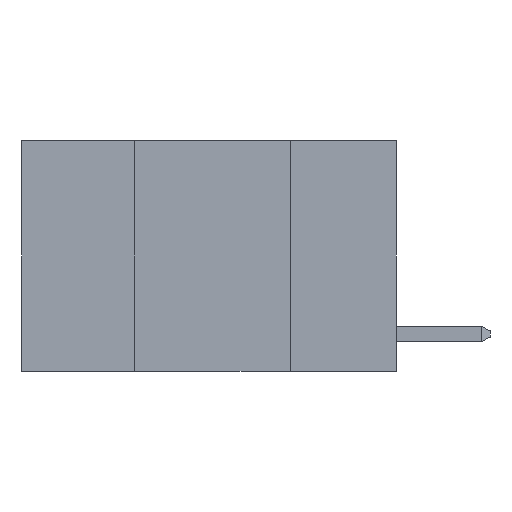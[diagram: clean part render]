
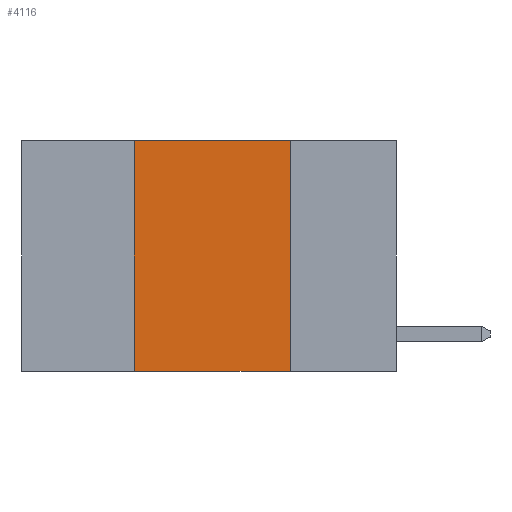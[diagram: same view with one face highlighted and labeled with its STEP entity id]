
A CAD part, left-side view. The second image highlights one B-rep face of the part: STEP entity #4116.
In plain terms, the highlighted planar face has unit normal (-1, 0, 0).
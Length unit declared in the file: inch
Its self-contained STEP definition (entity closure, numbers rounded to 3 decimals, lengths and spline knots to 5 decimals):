
#131 = CARTESIAN_POINT ( 'NONE',  ( 0., 0.17, -0.37 ) ) ;
#200 = LINE ( 'NONE', #8275, #9379 ) ;
#227 = DIRECTION ( 'NONE',  ( 0., 0., -1. ) ) ;
#299 = ORIENTED_EDGE ( 'NONE', *, *, #9837, .T. ) ;
#1164 = DIRECTION ( 'NONE',  ( 0., 0., -1. ) ) ;
#1300 = ORIENTED_EDGE ( 'NONE', *, *, #8317, .F. ) ;
#1396 = VERTEX_POINT ( 'NONE', #131 ) ;
#1507 = VECTOR ( 'NONE', #2159, 39.37008 ) ;
#1514 = AXIS2_PLACEMENT_3D ( 'NONE', #10785, #5665, #227 ) ;
#2061 = LINE ( 'NONE', #10009, #11068 ) ;
#2159 = DIRECTION ( 'NONE',  ( 0., -1., 0. ) ) ;
#2269 = FACE_OUTER_BOUND ( 'NONE', #3120, .T. ) ;
#2635 = CARTESIAN_POINT ( 'NONE',  ( 0., 0.17, 0. ) ) ;
#2678 = LINE ( 'NONE', #3634, #7139 ) ;
#3043 = DIRECTION ( 'NONE',  ( 0., 0., 1. ) ) ;
#3081 = CARTESIAN_POINT ( 'NONE',  ( 0., 0.6, -0.37 ) ) ;
#3120 = EDGE_LOOP ( 'NONE', ( #3880, #1300, #10405, #299 ) ) ;
#3579 = VERTEX_POINT ( 'NONE', #6548 ) ;
#3634 = CARTESIAN_POINT ( 'NONE',  ( 0., 0.6, 0. ) ) ;
#3880 = ORIENTED_EDGE ( 'NONE', *, *, #9771, .F. ) ;
#3938 = VERTEX_POINT ( 'NONE', #9627 ) ;
#4116 = ADVANCED_FACE ( 'NONE', ( #2269 ), #4756, .F. ) ;
#4756 = PLANE ( 'NONE',  #1514 ) ;
#5665 = DIRECTION ( 'NONE',  ( 1., 0., 0. ) ) ;
#6544 = LINE ( 'NONE', #3081, #1507 ) ;
#6548 = CARTESIAN_POINT ( 'NONE',  ( 0., 0.42, -0.37 ) ) ;
#7139 = VECTOR ( 'NONE', #8021, 39.37008 ) ;
#7187 = VERTEX_POINT ( 'NONE', #2635 ) ;
#8021 = DIRECTION ( 'NONE',  ( 0., -1., 0. ) ) ;
#8275 = CARTESIAN_POINT ( 'NONE',  ( 0., 0.17, 0. ) ) ;
#8317 = EDGE_CURVE ( 'NONE', #3938, #7187, #2678, .T. ) ;
#9379 = VECTOR ( 'NONE', #1164, 39.37008 ) ;
#9627 = CARTESIAN_POINT ( 'NONE',  ( 0., 0.42, 0. ) ) ;
#9771 = EDGE_CURVE ( 'NONE', #7187, #1396, #200, .T. ) ;
#9805 = EDGE_CURVE ( 'NONE', #3579, #3938, #2061, .T. ) ;
#9837 = EDGE_CURVE ( 'NONE', #3579, #1396, #6544, .T. ) ;
#10009 = CARTESIAN_POINT ( 'NONE',  ( 0., 0.42, 0. ) ) ;
#10405 = ORIENTED_EDGE ( 'NONE', *, *, #9805, .F. ) ;
#10785 = CARTESIAN_POINT ( 'NONE',  ( 0., 0.6, 0. ) ) ;
#11068 = VECTOR ( 'NONE', #3043, 39.37008 ) ;
